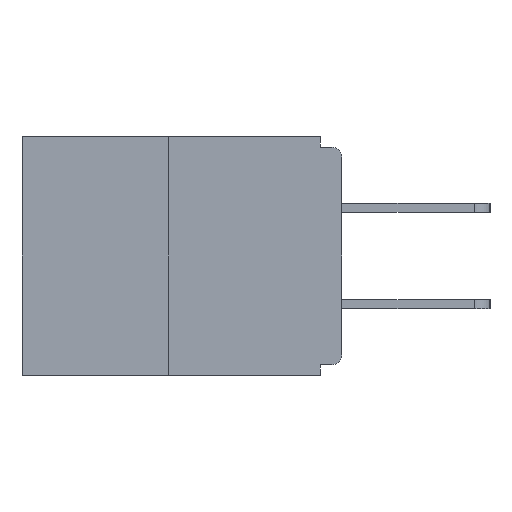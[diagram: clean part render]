
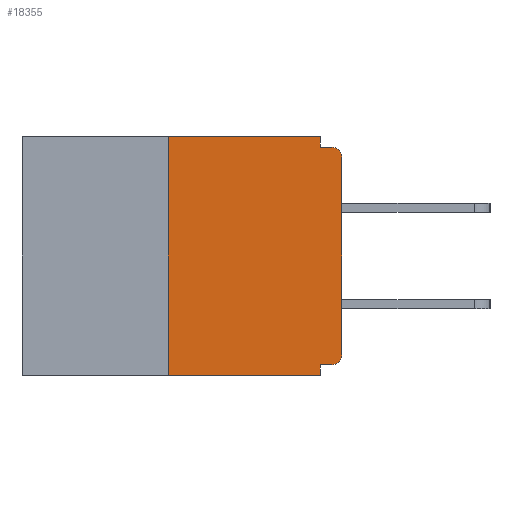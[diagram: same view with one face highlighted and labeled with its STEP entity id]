
A CAD part, left-side view. The second image highlights one B-rep face of the part: STEP entity #18355.
In plain terms, the highlighted planar face has unit normal (-1, 0, 0).
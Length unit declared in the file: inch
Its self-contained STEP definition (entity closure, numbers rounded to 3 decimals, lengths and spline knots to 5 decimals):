
#19 = CARTESIAN_POINT ( 'NONE',  ( 0., 0., 0. ) ) ;
#551 = LINE ( 'NONE', #2310, #12891 ) ;
#732 = EDGE_CURVE ( 'NONE', #20034, #12396, #8627, .T. ) ;
#818 = LINE ( 'NONE', #9423, #6397 ) ;
#908 = ORIENTED_EDGE ( 'NONE', *, *, #22248, .F. ) ;
#1561 = CARTESIAN_POINT ( 'NONE',  ( 0., 0., -0.313 ) ) ;
#2208 = DIRECTION ( 'NONE',  ( -1., 0., 0. ) ) ;
#2310 = CARTESIAN_POINT ( 'NONE',  ( 0., 0., -0.328 ) ) ;
#2373 = VECTOR ( 'NONE', #22591, 39.37008 ) ;
#2619 = CARTESIAN_POINT ( 'NONE',  ( 0., 0.015, -0.328 ) ) ;
#2796 = DIRECTION ( 'NONE',  ( 0., -1., 0. ) ) ;
#2966 = DIRECTION ( 'NONE',  ( -1., 0., 0. ) ) ;
#3346 = EDGE_CURVE ( 'NONE', #10992, #12396, #25325, .T. ) ;
#3561 = VECTOR ( 'NONE', #16490, 39.37008 ) ;
#3658 = ORIENTED_EDGE ( 'NONE', *, *, #6917, .T. ) ;
#3899 = AXIS2_PLACEMENT_3D ( 'NONE', #12403, #2208, #10393 ) ;
#4229 = PLANE ( 'NONE',  #9323 ) ;
#4363 = VERTEX_POINT ( 'NONE', #17664 ) ;
#4364 = DIRECTION ( 'NONE',  ( 0., 0., -1. ) ) ;
#4862 = DIRECTION ( 'NONE',  ( 0., -1., 0. ) ) ;
#5140 = CARTESIAN_POINT ( 'NONE',  ( 0., 0.031, -0.015 ) ) ;
#5146 = VERTEX_POINT ( 'NONE', #8612 ) ;
#5898 = LINE ( 'NONE', #20422, #19825 ) ;
#6139 = CARTESIAN_POINT ( 'NONE',  ( 0., 0.46, -0.343 ) ) ;
#6397 = VECTOR ( 'NONE', #17328, 39.37008 ) ;
#6790 = VERTEX_POINT ( 'NONE', #7916 ) ;
#6917 = EDGE_CURVE ( 'NONE', #4363, #26144, #22677, .T. ) ;
#7182 = DIRECTION ( 'NONE',  ( 0., 0., 1. ) ) ;
#7356 = EDGE_LOOP ( 'NONE', ( #16046, #11170, #3658, #18606, #16603, #12733, #20852, #19816, #17856, #908 ) ) ;
#7916 = CARTESIAN_POINT ( 'NONE',  ( 0., 0.25, 0. ) ) ;
#7933 = VECTOR ( 'NONE', #2796, 39.37008 ) ;
#8612 = CARTESIAN_POINT ( 'NONE',  ( 0., 0.031, 0. ) ) ;
#8627 = CIRCLE ( 'NONE', #3899, 0.015 ) ;
#9323 = AXIS2_PLACEMENT_3D ( 'NONE', #12431, #18607, #4364 ) ;
#9423 = CARTESIAN_POINT ( 'NONE',  ( 0., 0.031, -0.343 ) ) ;
#9712 = EDGE_CURVE ( 'NONE', #4363, #6790, #17761, .T. ) ;
#10336 = DIRECTION ( 'NONE',  ( 0., 0., -1. ) ) ;
#10393 = DIRECTION ( 'NONE',  ( 0., 0., -1. ) ) ;
#10992 = VERTEX_POINT ( 'NONE', #5140 ) ;
#11170 = ORIENTED_EDGE ( 'NONE', *, *, #9712, .F. ) ;
#12396 = VERTEX_POINT ( 'NONE', #21488 ) ;
#12403 = CARTESIAN_POINT ( 'NONE',  ( 0., 0.015, -0.03 ) ) ;
#12431 = CARTESIAN_POINT ( 'NONE',  ( 0., 0.46, 0. ) ) ;
#12733 = ORIENTED_EDGE ( 'NONE', *, *, #16458, .T. ) ;
#12891 = VECTOR ( 'NONE', #20832, 39.37008 ) ;
#13295 = CARTESIAN_POINT ( 'NONE',  ( 0., 0.015, -0.313 ) ) ;
#13458 = VERTEX_POINT ( 'NONE', #24109 ) ;
#14680 = CARTESIAN_POINT ( 'NONE',  ( 0., 0., -0.015 ) ) ;
#14881 = CARTESIAN_POINT ( 'NONE',  ( 0., 0.031, -0.343 ) ) ;
#15027 = DIRECTION ( 'NONE',  ( 0., 0., -1. ) ) ;
#15651 = EDGE_CURVE ( 'NONE', #6790, #5146, #21460, .T. ) ;
#16046 = ORIENTED_EDGE ( 'NONE', *, *, #15651, .F. ) ;
#16088 = CIRCLE ( 'NONE', #21682, 0.015 ) ;
#16322 = EDGE_CURVE ( 'NONE', #24918, #20034, #24869, .T. ) ;
#16458 = EDGE_CURVE ( 'NONE', #26356, #24918, #16088, .T. ) ;
#16490 = DIRECTION ( 'NONE',  ( 0., -1., 0. ) ) ;
#16603 = ORIENTED_EDGE ( 'NONE', *, *, #20892, .F. ) ;
#17328 = DIRECTION ( 'NONE',  ( 0., 0., -1. ) ) ;
#17494 = VECTOR ( 'NONE', #4862, 39.37008 ) ;
#17664 = CARTESIAN_POINT ( 'NONE',  ( 0., 0.25, -0.343 ) ) ;
#17716 = CARTESIAN_POINT ( 'NONE',  ( 0., 0., -0.03 ) ) ;
#17761 = LINE ( 'NONE', #23967, #25527 ) ;
#17856 = ORIENTED_EDGE ( 'NONE', *, *, #3346, .F. ) ;
#18355 = ADVANCED_FACE ( 'NONE', ( #20631 ), #4229, .F. ) ;
#18606 = ORIENTED_EDGE ( 'NONE', *, *, #19284, .F. ) ;
#18607 = DIRECTION ( 'NONE',  ( 1., 0., 0. ) ) ;
#19284 = EDGE_CURVE ( 'NONE', #13458, #26144, #818, .T. ) ;
#19299 = CARTESIAN_POINT ( 'NONE',  ( 0., 0.46, 0. ) ) ;
#19816 = ORIENTED_EDGE ( 'NONE', *, *, #732, .T. ) ;
#19825 = VECTOR ( 'NONE', #10336, 39.37008 ) ;
#20034 = VERTEX_POINT ( 'NONE', #17716 ) ;
#20422 = CARTESIAN_POINT ( 'NONE',  ( 0., 0.031, 0. ) ) ;
#20631 = FACE_OUTER_BOUND ( 'NONE', #7356, .T. ) ;
#20832 = DIRECTION ( 'NONE',  ( 0., 1., 0. ) ) ;
#20852 = ORIENTED_EDGE ( 'NONE', *, *, #16322, .T. ) ;
#20892 = EDGE_CURVE ( 'NONE', #26356, #13458, #551, .T. ) ;
#21460 = LINE ( 'NONE', #19299, #7933 ) ;
#21488 = CARTESIAN_POINT ( 'NONE',  ( 0., 0.015, -0.015 ) ) ;
#21682 = AXIS2_PLACEMENT_3D ( 'NONE', #13295, #2966, #15027 ) ;
#22248 = EDGE_CURVE ( 'NONE', #5146, #10992, #5898, .T. ) ;
#22591 = DIRECTION ( 'NONE',  ( 0., 0., 1. ) ) ;
#22677 = LINE ( 'NONE', #6139, #3561 ) ;
#23967 = CARTESIAN_POINT ( 'NONE',  ( 0., 0.25, 0. ) ) ;
#24109 = CARTESIAN_POINT ( 'NONE',  ( 0., 0.031, -0.328 ) ) ;
#24869 = LINE ( 'NONE', #19, #2373 ) ;
#24918 = VERTEX_POINT ( 'NONE', #1561 ) ;
#25325 = LINE ( 'NONE', #14680, #17494 ) ;
#25527 = VECTOR ( 'NONE', #7182, 39.37008 ) ;
#26144 = VERTEX_POINT ( 'NONE', #14881 ) ;
#26356 = VERTEX_POINT ( 'NONE', #2619 ) ;
